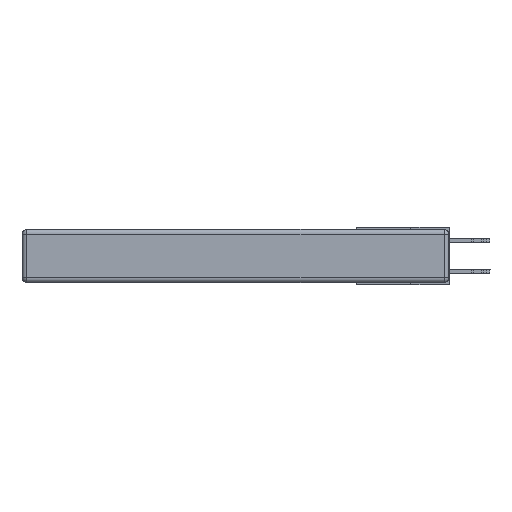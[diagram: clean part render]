
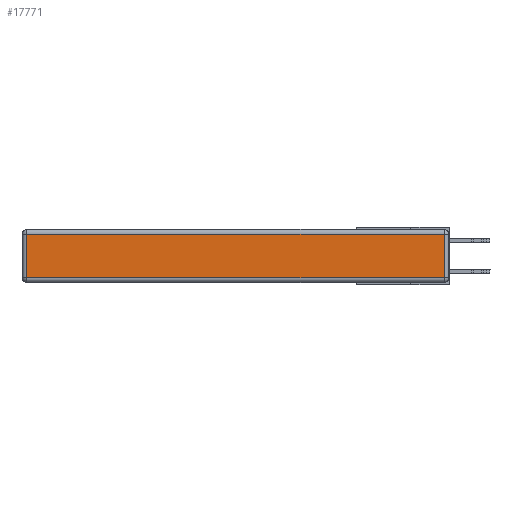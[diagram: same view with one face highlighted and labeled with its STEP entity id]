
A CAD part, left-side view. The second image highlights one B-rep face of the part: STEP entity #17771.
In plain terms, the highlighted planar face has unit normal (-1, 0, 0).
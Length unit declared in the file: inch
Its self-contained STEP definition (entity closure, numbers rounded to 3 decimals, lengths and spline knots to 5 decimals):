
#118 = CARTESIAN_POINT ( 'NONE',  ( 0., 0., -0.313 ) ) ;
#422 = VERTEX_POINT ( 'NONE', #1663 ) ;
#842 = DIRECTION ( 'NONE',  ( 0., 0., 1. ) ) ;
#988 = EDGE_CURVE ( 'NONE', #17666, #15572, #34183, .T. ) ;
#1663 = CARTESIAN_POINT ( 'NONE',  ( 0., 0.03, -0.03 ) ) ;
#3819 = LINE ( 'NONE', #12901, #21656 ) ;
#4245 = VECTOR ( 'NONE', #29181, 39.37008 ) ;
#5700 = VECTOR ( 'NONE', #842, 39.37008 ) ;
#7171 = AXIS2_PLACEMENT_3D ( 'NONE', #33103, #16559, #19328 ) ;
#8118 = DIRECTION ( 'NONE',  ( 0., 1., 0. ) ) ;
#8995 = CARTESIAN_POINT ( 'NONE',  ( 0., 0.03, -0.343 ) ) ;
#9078 = CARTESIAN_POINT ( 'NONE',  ( 0., 0.03, -0.313 ) ) ;
#9146 = ORIENTED_EDGE ( 'NONE', *, *, #34961, .T. ) ;
#9912 = LINE ( 'NONE', #16644, #30701 ) ;
#12901 = CARTESIAN_POINT ( 'NONE',  ( 0., 2.72, -0.343 ) ) ;
#15281 = EDGE_CURVE ( 'NONE', #422, #16134, #9912, .T. ) ;
#15572 = VERTEX_POINT ( 'NONE', #9078 ) ;
#16134 = VERTEX_POINT ( 'NONE', #18756 ) ;
#16559 = DIRECTION ( 'NONE',  ( -1., 0., 0. ) ) ;
#16644 = CARTESIAN_POINT ( 'NONE',  ( 0., 2.75, -0.03 ) ) ;
#17304 = ORIENTED_EDGE ( 'NONE', *, *, #988, .T. ) ;
#17666 = VERTEX_POINT ( 'NONE', #26758 ) ;
#17771 = ADVANCED_FACE ( 'NONE', ( #25398 ), #30310, .T. ) ;
#17850 = LINE ( 'NONE', #8995, #5700 ) ;
#18756 = CARTESIAN_POINT ( 'NONE',  ( 0., 2.72, -0.03 ) ) ;
#18912 = ORIENTED_EDGE ( 'NONE', *, *, #15281, .T. ) ;
#19328 = DIRECTION ( 'NONE',  ( 0., 0., 1. ) ) ;
#21656 = VECTOR ( 'NONE', #29460, 39.37008 ) ;
#22335 = EDGE_CURVE ( 'NONE', #16134, #17666, #3819, .T. ) ;
#22968 = ORIENTED_EDGE ( 'NONE', *, *, #22335, .T. ) ;
#25398 = FACE_OUTER_BOUND ( 'NONE', #29320, .T. ) ;
#26758 = CARTESIAN_POINT ( 'NONE',  ( 0., 2.72, -0.313 ) ) ;
#29181 = DIRECTION ( 'NONE',  ( 0., -1., 0. ) ) ;
#29320 = EDGE_LOOP ( 'NONE', ( #17304, #9146, #18912, #22968 ) ) ;
#29460 = DIRECTION ( 'NONE',  ( 0., 0., -1. ) ) ;
#30310 = PLANE ( 'NONE',  #7171 ) ;
#30701 = VECTOR ( 'NONE', #8118, 39.37008 ) ;
#33103 = CARTESIAN_POINT ( 'NONE',  ( 0., 0., -0.343 ) ) ;
#34183 = LINE ( 'NONE', #118, #4245 ) ;
#34961 = EDGE_CURVE ( 'NONE', #15572, #422, #17850, .T. ) ;
